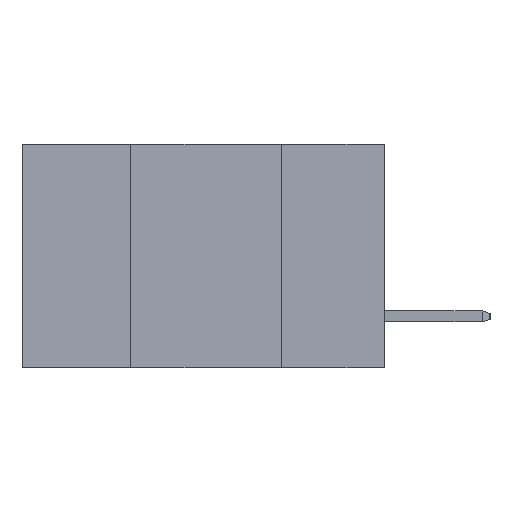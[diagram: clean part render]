
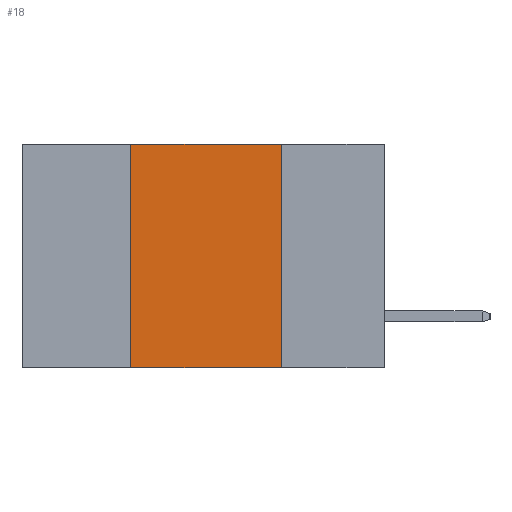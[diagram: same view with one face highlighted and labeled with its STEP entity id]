
A CAD part, left-side view. The second image highlights one B-rep face of the part: STEP entity #18.
In plain terms, the highlighted planar face has unit normal (-1, 0, 0).
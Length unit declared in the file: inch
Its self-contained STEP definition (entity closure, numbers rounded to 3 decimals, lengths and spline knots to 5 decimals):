
#18 = ADVANCED_FACE ( 'NONE', ( #4304 ), #4737, .F. ) ;
#824 = DIRECTION ( 'NONE',  ( 0., 0., 1. ) ) ;
#905 = LINE ( 'NONE', #2769, #12990 ) ;
#970 = VERTEX_POINT ( 'NONE', #18535 ) ;
#1172 = LINE ( 'NONE', #2267, #17998 ) ;
#2267 = CARTESIAN_POINT ( 'NONE',  ( 0., 0.17, -0.37 ) ) ;
#2485 = VERTEX_POINT ( 'NONE', #12372 ) ;
#2769 = CARTESIAN_POINT ( 'NONE',  ( 0., 0.42, -0.37 ) ) ;
#3234 = DIRECTION ( 'NONE',  ( 0., 0., -1. ) ) ;
#3388 = CARTESIAN_POINT ( 'NONE',  ( 0., 0.17, 0. ) ) ;
#3860 = EDGE_LOOP ( 'NONE', ( #13764, #14775, #18923, #6734 ) ) ;
#4304 = FACE_OUTER_BOUND ( 'NONE', #3860, .T. ) ;
#4737 = PLANE ( 'NONE',  #9697 ) ;
#5364 = CARTESIAN_POINT ( 'NONE',  ( 0., 0.6, 0. ) ) ;
#5536 = DIRECTION ( 'NONE',  ( 1., 0., 0. ) ) ;
#6308 = EDGE_CURVE ( 'NONE', #970, #2485, #11771, .T. ) ;
#6734 = ORIENTED_EDGE ( 'NONE', *, *, #6308, .T. ) ;
#6790 = VERTEX_POINT ( 'NONE', #7390 ) ;
#7360 = EDGE_CURVE ( 'NONE', #970, #6790, #905, .T. ) ;
#7390 = CARTESIAN_POINT ( 'NONE',  ( 0., 0.42, 0. ) ) ;
#8462 = EDGE_CURVE ( 'NONE', #6790, #10160, #9969, .T. ) ;
#8518 = CARTESIAN_POINT ( 'NONE',  ( 0., 0.6, 0. ) ) ;
#9354 = DIRECTION ( 'NONE',  ( 0., -1., 0. ) ) ;
#9697 = AXIS2_PLACEMENT_3D ( 'NONE', #5364, #5536, #3234 ) ;
#9756 = CARTESIAN_POINT ( 'NONE',  ( 0., 0.6, -0.37 ) ) ;
#9969 = LINE ( 'NONE', #8518, #17949 ) ;
#10160 = VERTEX_POINT ( 'NONE', #3388 ) ;
#11771 = LINE ( 'NONE', #9756, #16075 ) ;
#12372 = CARTESIAN_POINT ( 'NONE',  ( 0., 0.17, -0.37 ) ) ;
#12990 = VECTOR ( 'NONE', #824, 39.37008 ) ;
#13340 = DIRECTION ( 'NONE',  ( 0., 0., -1. ) ) ;
#13354 = DIRECTION ( 'NONE',  ( 0., -1., 0. ) ) ;
#13764 = ORIENTED_EDGE ( 'NONE', *, *, #13830, .F. ) ;
#13830 = EDGE_CURVE ( 'NONE', #10160, #2485, #1172, .T. ) ;
#14775 = ORIENTED_EDGE ( 'NONE', *, *, #8462, .F. ) ;
#16075 = VECTOR ( 'NONE', #9354, 39.37008 ) ;
#17949 = VECTOR ( 'NONE', #13354, 39.37008 ) ;
#17998 = VECTOR ( 'NONE', #13340, 39.37008 ) ;
#18535 = CARTESIAN_POINT ( 'NONE',  ( 0., 0.42, -0.37 ) ) ;
#18923 = ORIENTED_EDGE ( 'NONE', *, *, #7360, .F. ) ;
